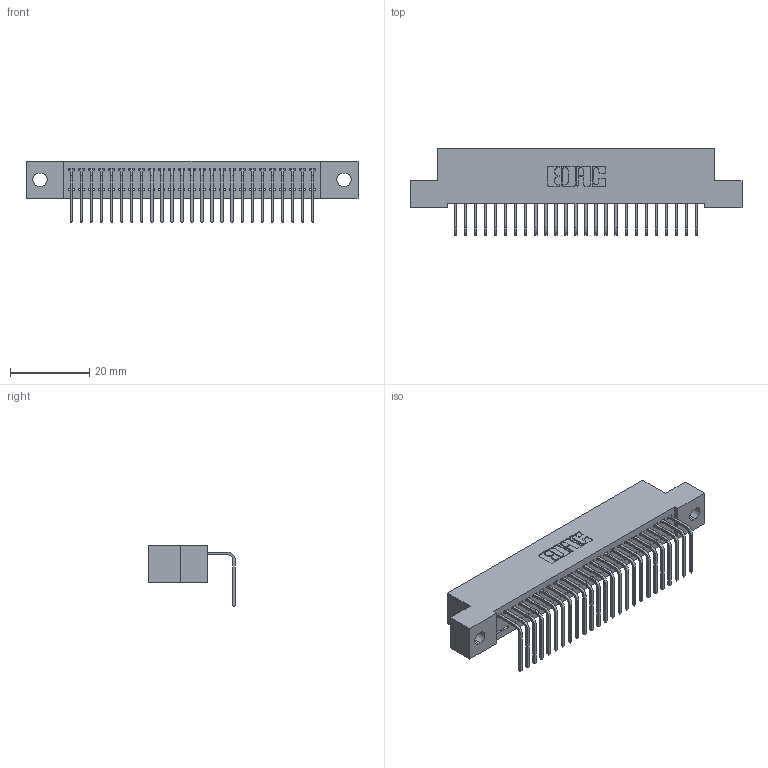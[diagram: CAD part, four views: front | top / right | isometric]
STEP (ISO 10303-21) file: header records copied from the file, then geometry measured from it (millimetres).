
FILE_DESCRIPTION (( 'STEP AP203' ), '1' );
FILE_NAME ('392-025-558-102.STEP', '2018-08-15T14:58:07', ( '' ), ( '' ), 'SwSTEP 2.0', 'SolidWorks 2016', '' );
FILE_SCHEMA (( 'CONFIG_CONTROL_DESIGN' ));
Length unit declared in the file: inch
Products named in the file (3): 342 Part_.128 Slot; 345-292-001_558 Tail - 2; 392-025-558-102
Assembly tree (26 placements, depth 2):
  392-025-558-102
    342 Part_.128 Slot
    345-292-001_558 Tail - 2  x25
Bounding box: 83.82 x 21.91 x 15.62 mm (x, y, z)
Volume: 7317.9 mm3; surface area: 10661.2 mm2
Topology: 26 solids, 26 shells, 1614 faces, 4861 edges, 3206 vertices
Faces by surface type: plane 1170, cylinder 444
Entity records: 17569 total; most frequent: CARTESIAN_POINT 3041, ORIENTED_EDGE 3002, DIRECTION 2599, EDGE_CURVE 1501, VECTOR 1373, LINE 1373, VERTEX_POINT 998, AXIS2_PLACEMENT_3D 613
